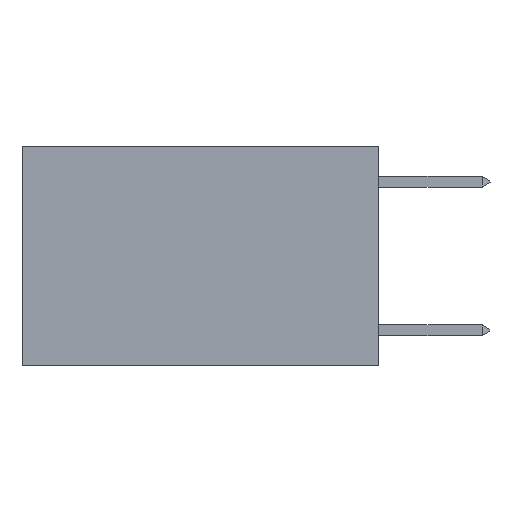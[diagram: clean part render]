
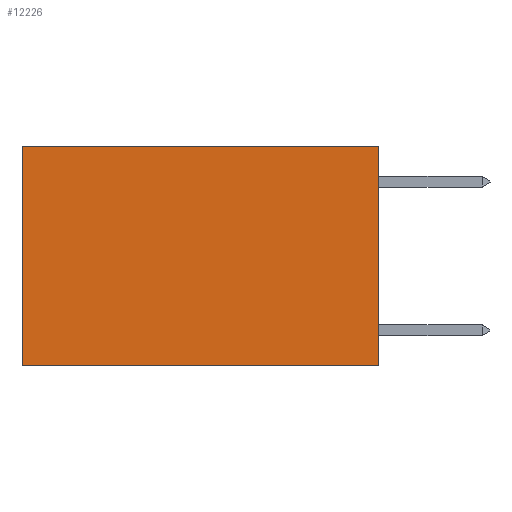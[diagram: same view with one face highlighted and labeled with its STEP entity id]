
A CAD part, left-side view. The second image highlights one B-rep face of the part: STEP entity #12226.
In plain terms, the highlighted planar face has unit normal (-1, 0, 0).
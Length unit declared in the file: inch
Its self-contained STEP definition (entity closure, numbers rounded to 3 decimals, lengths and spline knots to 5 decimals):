
#392 = ORIENTED_EDGE ( 'NONE', *, *, #13617, .T. ) ;
#1099 = FACE_OUTER_BOUND ( 'NONE', #6401, .T. ) ;
#2485 = PLANE ( 'NONE',  #18493 ) ;
#2990 = ORIENTED_EDGE ( 'NONE', *, *, #18546, .T. ) ;
#3396 = CARTESIAN_POINT ( 'NONE',  ( 0.2625, 0., 0. ) ) ;
#3580 = VERTEX_POINT ( 'NONE', #3747 ) ;
#3747 = CARTESIAN_POINT ( 'NONE',  ( 0.2625, 0., 0. ) ) ;
#4797 = LINE ( 'NONE', #6070, #12291 ) ;
#5006 = LINE ( 'NONE', #3396, #7377 ) ;
#5830 = VERTEX_POINT ( 'NONE', #14708 ) ;
#5993 = CARTESIAN_POINT ( 'NONE',  ( 0.2625, 0., 0. ) ) ;
#6070 = CARTESIAN_POINT ( 'NONE',  ( 0.2625, 0., 0. ) ) ;
#6401 = EDGE_LOOP ( 'NONE', ( #392, #18478, #11958, #2990 ) ) ;
#7154 = CARTESIAN_POINT ( 'NONE',  ( 0.2625, 0.6, 0. ) ) ;
#7377 = VECTOR ( 'NONE', #14934, 39.37008 ) ;
#7848 = EDGE_CURVE ( 'NONE', #3580, #5830, #4797, .T. ) ;
#7923 = EDGE_CURVE ( 'NONE', #5830, #9907, #19735, .T. ) ;
#9456 = CARTESIAN_POINT ( 'NONE',  ( 0.2625, 0.6, -0.37 ) ) ;
#9907 = VERTEX_POINT ( 'NONE', #9456 ) ;
#11707 = VECTOR ( 'NONE', #20425, 39.37008 ) ;
#11958 = ORIENTED_EDGE ( 'NONE', *, *, #7848, .F. ) ;
#11981 = VECTOR ( 'NONE', #13121, 39.37008 ) ;
#12226 = ADVANCED_FACE ( 'NONE', ( #1099 ), #2485, .F. ) ;
#12291 = VECTOR ( 'NONE', #12696, 39.37008 ) ;
#12696 = DIRECTION ( 'NONE',  ( 0., 0., -1. ) ) ;
#12749 = VERTEX_POINT ( 'NONE', #7154 ) ;
#13121 = DIRECTION ( 'NONE',  ( 0., 1., 0. ) ) ;
#13617 = EDGE_CURVE ( 'NONE', #12749, #9907, #14022, .T. ) ;
#14022 = LINE ( 'NONE', #18701, #11707 ) ;
#14708 = CARTESIAN_POINT ( 'NONE',  ( 0.2625, 0., -0.37 ) ) ;
#14934 = DIRECTION ( 'NONE',  ( 0., 1., 0. ) ) ;
#17088 = DIRECTION ( 'NONE',  ( 0., 0., -1. ) ) ;
#18114 = CARTESIAN_POINT ( 'NONE',  ( 0.2625, 0., -0.37 ) ) ;
#18478 = ORIENTED_EDGE ( 'NONE', *, *, #7923, .F. ) ;
#18493 = AXIS2_PLACEMENT_3D ( 'NONE', #5993, #18901, #17088 ) ;
#18546 = EDGE_CURVE ( 'NONE', #3580, #12749, #5006, .T. ) ;
#18701 = CARTESIAN_POINT ( 'NONE',  ( 0.2625, 0.6, 0. ) ) ;
#18901 = DIRECTION ( 'NONE',  ( 1., 0., 0. ) ) ;
#19735 = LINE ( 'NONE', #18114, #11981 ) ;
#20425 = DIRECTION ( 'NONE',  ( 0., 0., -1. ) ) ;
